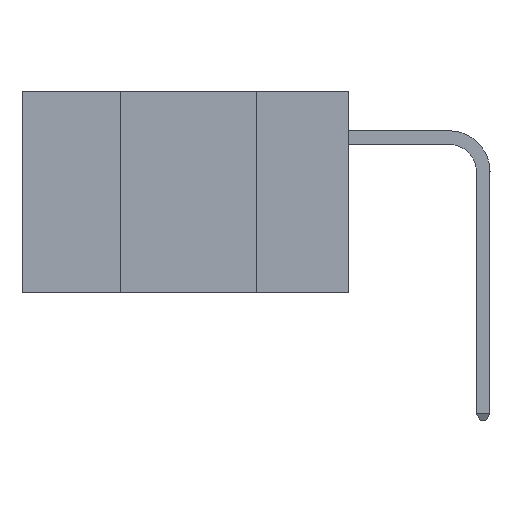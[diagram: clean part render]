
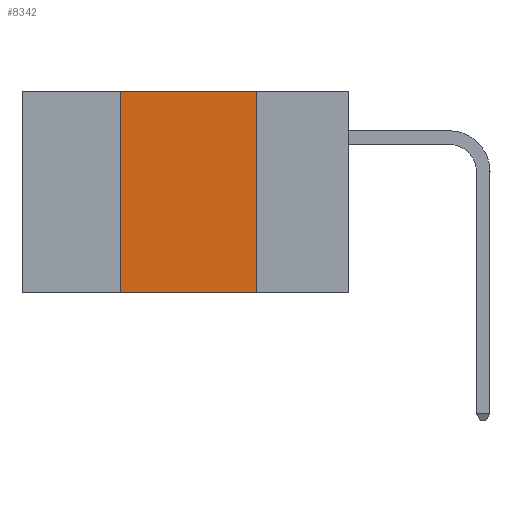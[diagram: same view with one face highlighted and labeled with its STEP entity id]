
A CAD part, left-side view. The second image highlights one B-rep face of the part: STEP entity #8342.
In plain terms, the highlighted planar face has unit normal (-1, 0, 0).
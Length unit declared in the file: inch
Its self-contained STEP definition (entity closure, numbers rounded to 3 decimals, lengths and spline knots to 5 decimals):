
#905 = ORIENTED_EDGE ( 'NONE', *, *, #11586, .F. ) ;
#1046 = PLANE ( 'NONE',  #11829 ) ;
#1509 = ORIENTED_EDGE ( 'NONE', *, *, #5690, .T. ) ;
#1925 = DIRECTION ( 'NONE',  ( 0., -1., 0. ) ) ;
#2545 = CARTESIAN_POINT ( 'NONE',  ( 0., 0.17, -0.37 ) ) ;
#3859 = CARTESIAN_POINT ( 'NONE',  ( 0., 0.42, -0.37 ) ) ;
#4255 = DIRECTION ( 'NONE',  ( 0., -1., 0. ) ) ;
#4341 = VERTEX_POINT ( 'NONE', #3859 ) ;
#5069 = CARTESIAN_POINT ( 'NONE',  ( 0., 0.42, 0. ) ) ;
#5323 = DIRECTION ( 'NONE',  ( 0., 0., -1. ) ) ;
#5690 = EDGE_CURVE ( 'NONE', #4341, #7278, #14606, .T. ) ;
#5895 = CARTESIAN_POINT ( 'NONE',  ( 0., 0.42, 0. ) ) ;
#6076 = DIRECTION ( 'NONE',  ( 1., 0., 0. ) ) ;
#6936 = VECTOR ( 'NONE', #1925, 39.37008 ) ;
#7278 = VERTEX_POINT ( 'NONE', #2545 ) ;
#7295 = EDGE_LOOP ( 'NONE', ( #905, #15152, #12811, #1509 ) ) ;
#7801 = LINE ( 'NONE', #5069, #11765 ) ;
#8342 = ADVANCED_FACE ( 'NONE', ( #12391 ), #1046, .F. ) ;
#8743 = DIRECTION ( 'NONE',  ( 0., 0., 1. ) ) ;
#9029 = CARTESIAN_POINT ( 'NONE',  ( 0., 0.17, 0. ) ) ;
#10817 = EDGE_CURVE ( 'NONE', #4341, #12523, #7801, .T. ) ;
#11586 = EDGE_CURVE ( 'NONE', #15115, #7278, #12100, .T. ) ;
#11734 = VECTOR ( 'NONE', #5323, 39.37008 ) ;
#11765 = VECTOR ( 'NONE', #8743, 39.37008 ) ;
#11829 = AXIS2_PLACEMENT_3D ( 'NONE', #13300, #6076, #14462 ) ;
#12100 = LINE ( 'NONE', #9029, #11734 ) ;
#12391 = FACE_OUTER_BOUND ( 'NONE', #7295, .T. ) ;
#12523 = VERTEX_POINT ( 'NONE', #5895 ) ;
#12774 = CARTESIAN_POINT ( 'NONE',  ( 0., 0.6, -0.37 ) ) ;
#12811 = ORIENTED_EDGE ( 'NONE', *, *, #10817, .F. ) ;
#13296 = LINE ( 'NONE', #15190, #6936 ) ;
#13300 = CARTESIAN_POINT ( 'NONE',  ( 0., 0.6, 0. ) ) ;
#14259 = VECTOR ( 'NONE', #4255, 39.37008 ) ;
#14455 = EDGE_CURVE ( 'NONE', #12523, #15115, #13296, .T. ) ;
#14462 = DIRECTION ( 'NONE',  ( 0., 0., -1. ) ) ;
#14606 = LINE ( 'NONE', #12774, #14259 ) ;
#15115 = VERTEX_POINT ( 'NONE', #15274 ) ;
#15152 = ORIENTED_EDGE ( 'NONE', *, *, #14455, .F. ) ;
#15190 = CARTESIAN_POINT ( 'NONE',  ( 0., 0.6, 0. ) ) ;
#15274 = CARTESIAN_POINT ( 'NONE',  ( 0., 0.17, 0. ) ) ;
